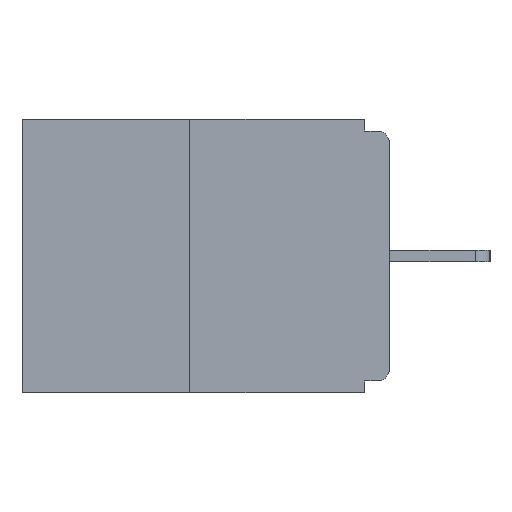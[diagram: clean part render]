
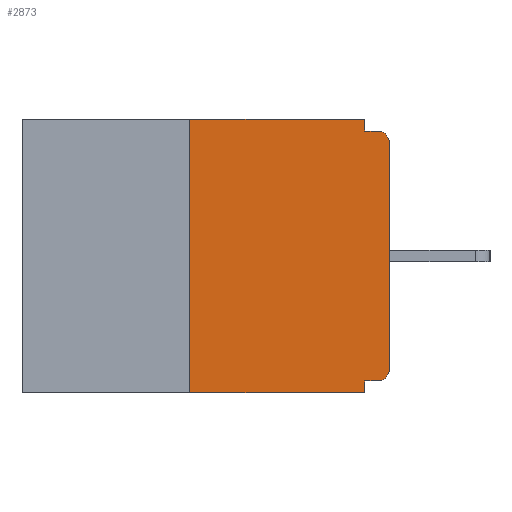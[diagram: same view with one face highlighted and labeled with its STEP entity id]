
A CAD part, left-side view. The second image highlights one B-rep face of the part: STEP entity #2873.
In plain terms, the highlighted planar face has unit normal (-1, 0, 0).
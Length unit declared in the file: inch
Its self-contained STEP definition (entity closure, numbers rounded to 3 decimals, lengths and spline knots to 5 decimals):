
#97 = CARTESIAN_POINT ( 'NONE',  ( 0., 0.031, -0.328 ) ) ;
#257 = CARTESIAN_POINT ( 'NONE',  ( 0., 0.015, -0.015 ) ) ;
#440 = DIRECTION ( 'NONE',  ( 0., -1., 0. ) ) ;
#1199 = VECTOR ( 'NONE', #8443, 39.37008 ) ;
#1247 = CIRCLE ( 'NONE', #4341, 0.015 ) ;
#1370 = DIRECTION ( 'NONE',  ( 0., 0., -1. ) ) ;
#1647 = LINE ( 'NONE', #13322, #8072 ) ;
#1840 = LINE ( 'NONE', #11636, #7247 ) ;
#2873 = ADVANCED_FACE ( 'NONE', ( #4350 ), #11379, .F. ) ;
#2888 = DIRECTION ( 'NONE',  ( 0., 0., -1. ) ) ;
#2946 = VERTEX_POINT ( 'NONE', #13698 ) ;
#3017 = CARTESIAN_POINT ( 'NONE',  ( 0., 0.015, -0.03 ) ) ;
#3267 = EDGE_CURVE ( 'NONE', #7280, #3677, #7647, .T. ) ;
#3619 = CARTESIAN_POINT ( 'NONE',  ( 0., 0.031, -0.343 ) ) ;
#3677 = VERTEX_POINT ( 'NONE', #12619 ) ;
#3926 = DIRECTION ( 'NONE',  ( 1., 0., 0. ) ) ;
#4166 = DIRECTION ( 'NONE',  ( 0., 0., -1. ) ) ;
#4170 = CARTESIAN_POINT ( 'NONE',  ( 0., 0.031, 0. ) ) ;
#4207 = DIRECTION ( 'NONE',  ( 0., 1., 0. ) ) ;
#4260 = EDGE_CURVE ( 'NONE', #11897, #10900, #10226, .T. ) ;
#4341 = AXIS2_PLACEMENT_3D ( 'NONE', #13859, #8228, #1370 ) ;
#4350 = FACE_OUTER_BOUND ( 'NONE', #4587, .T. ) ;
#4431 = DIRECTION ( 'NONE',  ( 0., 0., 1. ) ) ;
#4587 = EDGE_LOOP ( 'NONE', ( #13539, #12830, #12265, #13421, #11637, #11196, #12203, #13196, #12927, #13153 ) ) ;
#4701 = VECTOR ( 'NONE', #440, 39.37008 ) ;
#5283 = CARTESIAN_POINT ( 'NONE',  ( 0., 0., -0.328 ) ) ;
#5296 = DIRECTION ( 'NONE',  ( 0., 0., -1. ) ) ;
#5421 = CARTESIAN_POINT ( 'NONE',  ( 0., 0.25, 0. ) ) ;
#5881 = CARTESIAN_POINT ( 'NONE',  ( 0., 0., -0.313 ) ) ;
#6300 = CARTESIAN_POINT ( 'NONE',  ( 0., 0.46, 0. ) ) ;
#6305 = CARTESIAN_POINT ( 'NONE',  ( 0., 0.46, -0.343 ) ) ;
#6790 = EDGE_CURVE ( 'NONE', #10900, #10019, #7668, .T. ) ;
#6985 = CARTESIAN_POINT ( 'NONE',  ( 0., 0., 0. ) ) ;
#7202 = VERTEX_POINT ( 'NONE', #7475 ) ;
#7247 = VECTOR ( 'NONE', #4431, 39.37008 ) ;
#7280 = VERTEX_POINT ( 'NONE', #5421 ) ;
#7475 = CARTESIAN_POINT ( 'NONE',  ( 0., 0.25, -0.343 ) ) ;
#7562 = DIRECTION ( 'NONE',  ( 0., 0., 1. ) ) ;
#7611 = AXIS2_PLACEMENT_3D ( 'NONE', #11320, #3926, #2888 ) ;
#7647 = LINE ( 'NONE', #6300, #4701 ) ;
#7653 = CARTESIAN_POINT ( 'NONE',  ( 0., 0.031, -0.015 ) ) ;
#7668 = CIRCLE ( 'NONE', #11740, 0.015 ) ;
#7783 = VERTEX_POINT ( 'NONE', #11164 ) ;
#8072 = VECTOR ( 'NONE', #12399, 39.37008 ) ;
#8221 = VECTOR ( 'NONE', #11896, 39.37008 ) ;
#8228 = DIRECTION ( 'NONE',  ( -1., 0., 0. ) ) ;
#8396 = VECTOR ( 'NONE', #5296, 39.37008 ) ;
#8443 = DIRECTION ( 'NONE',  ( 0., -1., 0. ) ) ;
#8866 = EDGE_CURVE ( 'NONE', #2946, #11897, #1247, .T. ) ;
#9182 = CARTESIAN_POINT ( 'NONE',  ( 0., 0., -0.03 ) ) ;
#9437 = LINE ( 'NONE', #5283, #11694 ) ;
#9442 = VERTEX_POINT ( 'NONE', #7653 ) ;
#10019 = VERTEX_POINT ( 'NONE', #257 ) ;
#10052 = LINE ( 'NONE', #6305, #1199 ) ;
#10160 = EDGE_CURVE ( 'NONE', #9442, #10019, #1647, .T. ) ;
#10226 = LINE ( 'NONE', #6985, #12444 ) ;
#10453 = DIRECTION ( 'NONE',  ( -1., 0., 0. ) ) ;
#10900 = VERTEX_POINT ( 'NONE', #9182 ) ;
#11164 = CARTESIAN_POINT ( 'NONE',  ( 0., 0.031, -0.343 ) ) ;
#11196 = ORIENTED_EDGE ( 'NONE', *, *, #8866, .T. ) ;
#11277 = EDGE_CURVE ( 'NONE', #3677, #9442, #13695, .T. ) ;
#11320 = CARTESIAN_POINT ( 'NONE',  ( 0., 0.46, 0. ) ) ;
#11379 = PLANE ( 'NONE',  #7611 ) ;
#11636 = CARTESIAN_POINT ( 'NONE',  ( 0., 0.25, 0. ) ) ;
#11637 = ORIENTED_EDGE ( 'NONE', *, *, #12695, .F. ) ;
#11694 = VECTOR ( 'NONE', #4207, 39.37008 ) ;
#11740 = AXIS2_PLACEMENT_3D ( 'NONE', #3017, #10453, #4166 ) ;
#11896 = DIRECTION ( 'NONE',  ( 0., 0., -1. ) ) ;
#11897 = VERTEX_POINT ( 'NONE', #5881 ) ;
#11917 = EDGE_CURVE ( 'NONE', #12324, #7783, #13290, .T. ) ;
#12203 = ORIENTED_EDGE ( 'NONE', *, *, #4260, .T. ) ;
#12265 = ORIENTED_EDGE ( 'NONE', *, *, #12532, .T. ) ;
#12324 = VERTEX_POINT ( 'NONE', #97 ) ;
#12399 = DIRECTION ( 'NONE',  ( 0., -1., 0. ) ) ;
#12444 = VECTOR ( 'NONE', #7562, 39.37008 ) ;
#12532 = EDGE_CURVE ( 'NONE', #7202, #7783, #10052, .T. ) ;
#12619 = CARTESIAN_POINT ( 'NONE',  ( 0., 0.031, 0. ) ) ;
#12695 = EDGE_CURVE ( 'NONE', #2946, #12324, #9437, .T. ) ;
#12830 = ORIENTED_EDGE ( 'NONE', *, *, #13143, .F. ) ;
#12927 = ORIENTED_EDGE ( 'NONE', *, *, #10160, .F. ) ;
#13143 = EDGE_CURVE ( 'NONE', #7202, #7280, #1840, .T. ) ;
#13153 = ORIENTED_EDGE ( 'NONE', *, *, #11277, .F. ) ;
#13196 = ORIENTED_EDGE ( 'NONE', *, *, #6790, .T. ) ;
#13290 = LINE ( 'NONE', #3619, #8221 ) ;
#13322 = CARTESIAN_POINT ( 'NONE',  ( 0., 0., -0.015 ) ) ;
#13421 = ORIENTED_EDGE ( 'NONE', *, *, #11917, .F. ) ;
#13539 = ORIENTED_EDGE ( 'NONE', *, *, #3267, .F. ) ;
#13695 = LINE ( 'NONE', #4170, #8396 ) ;
#13698 = CARTESIAN_POINT ( 'NONE',  ( 0., 0.015, -0.328 ) ) ;
#13859 = CARTESIAN_POINT ( 'NONE',  ( 0., 0.015, -0.313 ) ) ;
